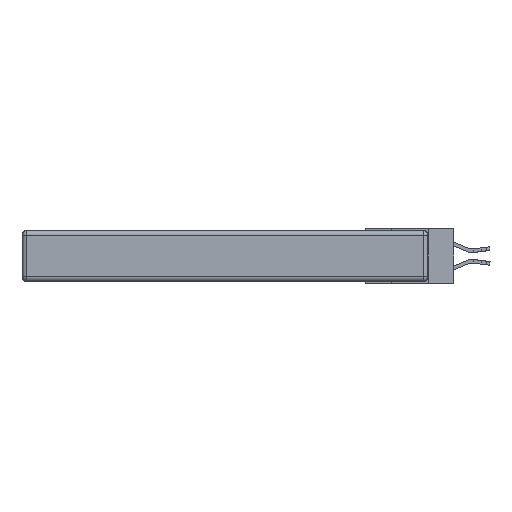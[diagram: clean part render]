
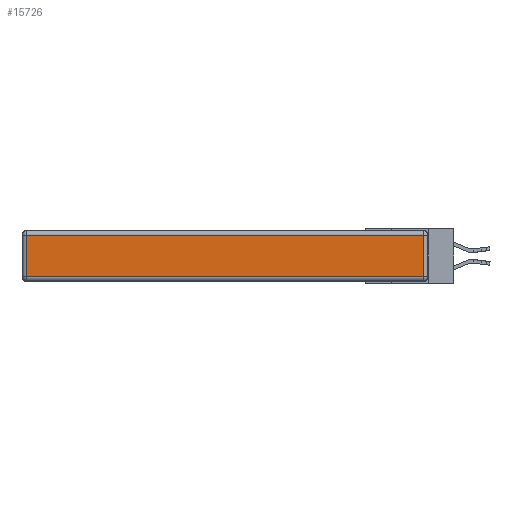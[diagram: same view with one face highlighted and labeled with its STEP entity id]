
A CAD part, left-side view. The second image highlights one B-rep face of the part: STEP entity #15726.
In plain terms, the highlighted planar face has unit normal (-1, 0, 0).
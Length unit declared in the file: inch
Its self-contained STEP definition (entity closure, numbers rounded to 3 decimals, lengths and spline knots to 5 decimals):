
#93 = LINE ( 'NONE', #15886, #18533 ) ;
#1756 = ORIENTED_EDGE ( 'NONE', *, *, #13909, .T. ) ;
#1818 = EDGE_CURVE ( 'NONE', #16854, #18639, #17427, .T. ) ;
#1926 = CARTESIAN_POINT ( 'NONE',  ( 0., 0.03, -0.03 ) ) ;
#1998 = DIRECTION ( 'NONE',  ( -1., 0., 0. ) ) ;
#2055 = VERTEX_POINT ( 'NONE', #13940 ) ;
#3526 = AXIS2_PLACEMENT_3D ( 'NONE', #11661, #1998, #19824 ) ;
#3579 = CARTESIAN_POINT ( 'NONE',  ( 0., 0.03, -0.343 ) ) ;
#4454 = EDGE_CURVE ( 'NONE', #6183, #16854, #93, .T. ) ;
#4885 = DIRECTION ( 'NONE',  ( 0., 1., 0. ) ) ;
#4982 = ORIENTED_EDGE ( 'NONE', *, *, #1818, .T. ) ;
#5040 = CARTESIAN_POINT ( 'NONE',  ( 0., 2.72, -0.343 ) ) ;
#5266 = VECTOR ( 'NONE', #13176, 39.37008 ) ;
#6183 = VERTEX_POINT ( 'NONE', #17108 ) ;
#6746 = CARTESIAN_POINT ( 'NONE',  ( 0., 0.03, -0.313 ) ) ;
#10866 = DIRECTION ( 'NONE',  ( 0., -1., 0. ) ) ;
#11065 = ORIENTED_EDGE ( 'NONE', *, *, #11715, .T. ) ;
#11432 = DIRECTION ( 'NONE',  ( 0., 0., -1. ) ) ;
#11550 = CARTESIAN_POINT ( 'NONE',  ( 0., 2.75, -0.03 ) ) ;
#11661 = CARTESIAN_POINT ( 'NONE',  ( 0., 0., -0.343 ) ) ;
#11715 = EDGE_CURVE ( 'NONE', #18639, #2055, #20140, .T. ) ;
#13065 = FACE_OUTER_BOUND ( 'NONE', #17858, .T. ) ;
#13176 = DIRECTION ( 'NONE',  ( 0., 0., 1. ) ) ;
#13909 = EDGE_CURVE ( 'NONE', #2055, #6183, #19531, .T. ) ;
#13940 = CARTESIAN_POINT ( 'NONE',  ( 0., 2.72, -0.03 ) ) ;
#15564 = ORIENTED_EDGE ( 'NONE', *, *, #4454, .T. ) ;
#15726 = ADVANCED_FACE ( 'NONE', ( #13065 ), #16746, .T. ) ;
#15886 = CARTESIAN_POINT ( 'NONE',  ( 0., 0., -0.313 ) ) ;
#16746 = PLANE ( 'NONE',  #3526 ) ;
#16854 = VERTEX_POINT ( 'NONE', #6746 ) ;
#17108 = CARTESIAN_POINT ( 'NONE',  ( 0., 2.72, -0.313 ) ) ;
#17427 = LINE ( 'NONE', #3579, #5266 ) ;
#17858 = EDGE_LOOP ( 'NONE', ( #15564, #4982, #11065, #1756 ) ) ;
#17963 = VECTOR ( 'NONE', #11432, 39.37008 ) ;
#18533 = VECTOR ( 'NONE', #10866, 39.37008 ) ;
#18639 = VERTEX_POINT ( 'NONE', #1926 ) ;
#19531 = LINE ( 'NONE', #5040, #17963 ) ;
#19628 = VECTOR ( 'NONE', #4885, 39.37008 ) ;
#19824 = DIRECTION ( 'NONE',  ( 0., 0., 1. ) ) ;
#20140 = LINE ( 'NONE', #11550, #19628 ) ;
